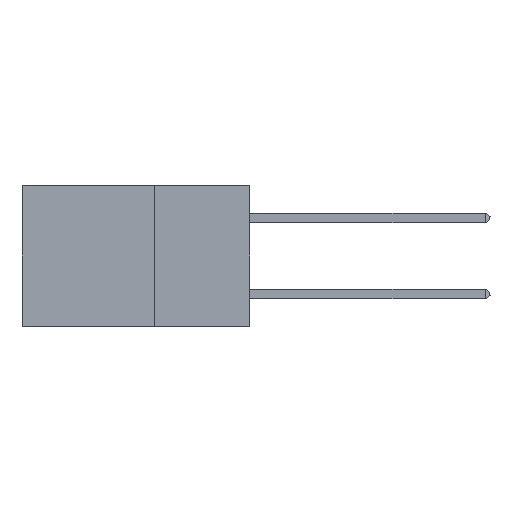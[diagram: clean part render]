
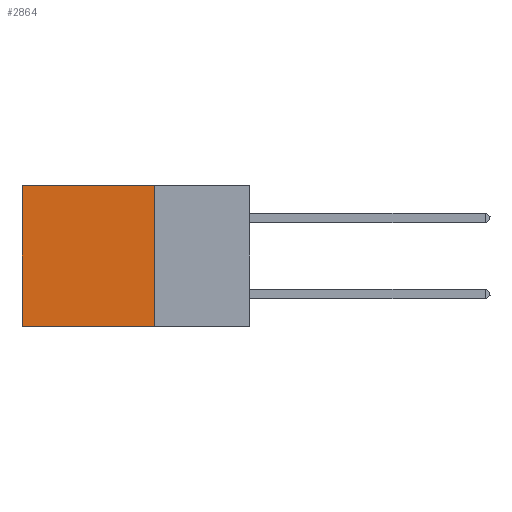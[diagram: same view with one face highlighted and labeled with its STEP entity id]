
A CAD part, left-side view. The second image highlights one B-rep face of the part: STEP entity #2864.
In plain terms, the highlighted planar face has unit normal (-1, 0, 0).
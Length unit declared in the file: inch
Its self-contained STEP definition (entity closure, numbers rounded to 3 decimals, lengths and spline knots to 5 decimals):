
#1245 = VERTEX_POINT ( 'NONE', #13866 ) ;
#1461 = VERTEX_POINT ( 'NONE', #20290 ) ;
#2291 = DIRECTION ( 'NONE',  ( 0., 1., 0. ) ) ;
#2398 = LINE ( 'NONE', #29460, #22940 ) ;
#2602 = ORIENTED_EDGE ( 'NONE', *, *, #20441, .T. ) ;
#2864 = ADVANCED_FACE ( 'NONE', ( #15950 ), #11944, .F. ) ;
#3316 = ORIENTED_EDGE ( 'NONE', *, *, #15102, .T. ) ;
#7600 = EDGE_LOOP ( 'NONE', ( #2602, #26287, #8061, #3316 ) ) ;
#8061 = ORIENTED_EDGE ( 'NONE', *, *, #15260, .F. ) ;
#8102 = CARTESIAN_POINT ( 'NONE',  ( 0.2875, 0.6, 0. ) ) ;
#8661 = CARTESIAN_POINT ( 'NONE',  ( 0.2875, 0.25, 0. ) ) ;
#10820 = CARTESIAN_POINT ( 'NONE',  ( 0.2875, 0.25, 0. ) ) ;
#11944 = PLANE ( 'NONE',  #34693 ) ;
#13866 = CARTESIAN_POINT ( 'NONE',  ( 0.2875, 0.25, -0.37 ) ) ;
#14360 = CARTESIAN_POINT ( 'NONE',  ( 0.2875, 0.25, -0.37 ) ) ;
#14734 = DIRECTION ( 'NONE',  ( 1., 0., 0. ) ) ;
#15102 = EDGE_CURVE ( 'NONE', #1461, #33290, #18571, .T. ) ;
#15260 = EDGE_CURVE ( 'NONE', #1461, #1245, #34555, .T. ) ;
#15950 = FACE_OUTER_BOUND ( 'NONE', #7600, .T. ) ;
#18571 = LINE ( 'NONE', #10820, #32392 ) ;
#19798 = DIRECTION ( 'NONE',  ( 0., 0., -1. ) ) ;
#20290 = CARTESIAN_POINT ( 'NONE',  ( 0.2875, 0.25, 0. ) ) ;
#20441 = EDGE_CURVE ( 'NONE', #33290, #34721, #2398, .T. ) ;
#22940 = VECTOR ( 'NONE', #32233, 39.37008 ) ;
#24764 = LINE ( 'NONE', #14360, #31279 ) ;
#26287 = ORIENTED_EDGE ( 'NONE', *, *, #34024, .F. ) ;
#27171 = VECTOR ( 'NONE', #19798, 39.37008 ) ;
#29460 = CARTESIAN_POINT ( 'NONE',  ( 0.2875, 0.6, 0. ) ) ;
#30996 = CARTESIAN_POINT ( 'NONE',  ( 0.2875, 0.6, -0.37 ) ) ;
#31279 = VECTOR ( 'NONE', #33699, 39.37008 ) ;
#31303 = CARTESIAN_POINT ( 'NONE',  ( 0.2875, 0.25, 0. ) ) ;
#32233 = DIRECTION ( 'NONE',  ( 0., 0., -1. ) ) ;
#32392 = VECTOR ( 'NONE', #2291, 39.37008 ) ;
#33290 = VERTEX_POINT ( 'NONE', #8102 ) ;
#33699 = DIRECTION ( 'NONE',  ( 0., 1., 0. ) ) ;
#34024 = EDGE_CURVE ( 'NONE', #1245, #34721, #24764, .T. ) ;
#34081 = DIRECTION ( 'NONE',  ( 0., 0., -1. ) ) ;
#34555 = LINE ( 'NONE', #8661, #27171 ) ;
#34693 = AXIS2_PLACEMENT_3D ( 'NONE', #31303, #14734, #34081 ) ;
#34721 = VERTEX_POINT ( 'NONE', #30996 ) ;
